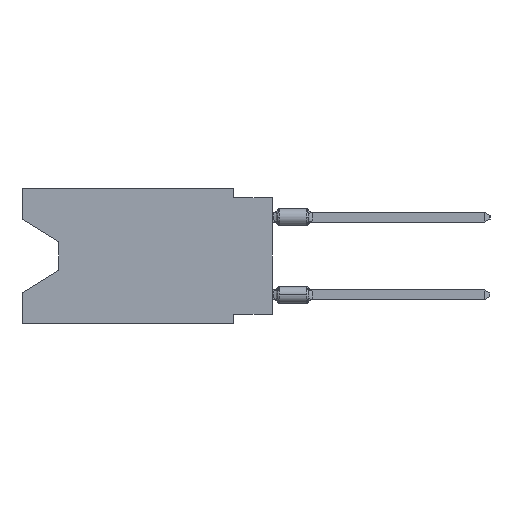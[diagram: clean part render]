
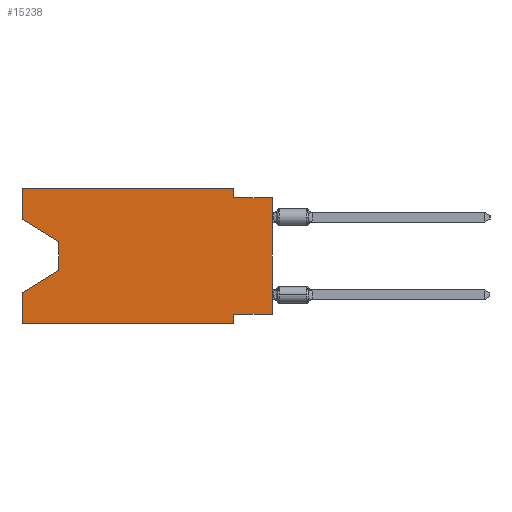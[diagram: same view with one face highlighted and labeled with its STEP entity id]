
A CAD part, left-side view. The second image highlights one B-rep face of the part: STEP entity #15238.
In plain terms, the highlighted planar face has unit normal (-1, 0, 0).
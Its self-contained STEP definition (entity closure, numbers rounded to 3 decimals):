
#45 = CARTESIAN_POINT ( 'NONE',  ( 0., 16.383, 0. ) ) ;
#332 = LINE ( 'NONE', #27026, #490 ) ;
#490 = VECTOR ( 'NONE', #9860, 1000. ) ;
#760 = LINE ( 'NONE', #24597, #28645 ) ;
#1289 = DIRECTION ( 'NONE',  ( 0., -1., 0. ) ) ;
#1297 = VERTEX_POINT ( 'NONE', #8697 ) ;
#1595 = VERTEX_POINT ( 'NONE', #38771 ) ;
#2137 = CARTESIAN_POINT ( 'NONE',  ( 0., 2.54, -8.255 ) ) ;
#2573 = CARTESIAN_POINT ( 'NONE',  ( 0., 13.97, -3.505 ) ) ;
#2845 = EDGE_CURVE ( 'NONE', #24659, #15315, #19701, .T. ) ;
#3025 = DIRECTION ( 'NONE',  ( 0., 0., -1. ) ) ;
#3089 = AXIS2_PLACEMENT_3D ( 'NONE', #24086, #35317, #35539 ) ;
#3456 = ORIENTED_EDGE ( 'NONE', *, *, #19535, .F. ) ;
#3770 = EDGE_CURVE ( 'NONE', #29179, #15438, #28656, .T. ) ;
#4146 = VERTEX_POINT ( 'NONE', #2573 ) ;
#4383 = ORIENTED_EDGE ( 'NONE', *, *, #30460, .F. ) ;
#5077 = FACE_OUTER_BOUND ( 'NONE', #12166, .T. ) ;
#5600 = CARTESIAN_POINT ( 'NONE',  ( 0., 0., 0. ) ) ;
#5640 = EDGE_CURVE ( 'NONE', #15473, #15072, #760, .T. ) ;
#5659 = VECTOR ( 'NONE', #24197, 1000. ) ;
#6470 = ORIENTED_EDGE ( 'NONE', *, *, #36871, .F. ) ;
#6519 = CARTESIAN_POINT ( 'NONE',  ( 0., 13.97, -5.385 ) ) ;
#7117 = VERTEX_POINT ( 'NONE', #41844 ) ;
#7897 = LINE ( 'NONE', #42127, #26579 ) ;
#8697 = CARTESIAN_POINT ( 'NONE',  ( 0., 0., -0.635 ) ) ;
#9201 = EDGE_CURVE ( 'NONE', #7117, #1297, #18195, .T. ) ;
#9860 = DIRECTION ( 'NONE',  ( 0., -1., 0. ) ) ;
#10411 = ORIENTED_EDGE ( 'NONE', *, *, #14484, .F. ) ;
#10516 = CARTESIAN_POINT ( 'NONE',  ( 0., 0., -8.255 ) ) ;
#10759 = CARTESIAN_POINT ( 'NONE',  ( 0., 16.383, -2.038 ) ) ;
#10935 = DIRECTION ( 'NONE',  ( 0., -1., 0. ) ) ;
#11017 = CARTESIAN_POINT ( 'NONE',  ( 0., 16.383, -8.89 ) ) ;
#12166 = EDGE_LOOP ( 'NONE', ( #20051, #15678, #16820, #41837, #31836, #3456, #4383, #42537, #16226, #40885, #10411, #6470 ) ) ;
#13141 = CARTESIAN_POINT ( 'NONE',  ( 0., 16.383, 0. ) ) ;
#14484 = EDGE_CURVE ( 'NONE', #18626, #24659, #7897, .T. ) ;
#14534 = VECTOR ( 'NONE', #32481, 1000. ) ;
#15072 = VERTEX_POINT ( 'NONE', #17059 ) ;
#15238 = ADVANCED_FACE ( 'NONE', ( #5077 ), #32442, .F. ) ;
#15315 = VERTEX_POINT ( 'NONE', #26036 ) ;
#15438 = VERTEX_POINT ( 'NONE', #39933 ) ;
#15473 = VERTEX_POINT ( 'NONE', #11017 ) ;
#15678 = ORIENTED_EDGE ( 'NONE', *, *, #30527, .T. ) ;
#15765 = CARTESIAN_POINT ( 'NONE',  ( 0., 2.54, 0. ) ) ;
#16226 = ORIENTED_EDGE ( 'NONE', *, *, #38185, .F. ) ;
#16489 = CARTESIAN_POINT ( 'NONE',  ( 0., 13.97, -3.505 ) ) ;
#16645 = CARTESIAN_POINT ( 'NONE',  ( 0., 2.54, -8.89 ) ) ;
#16820 = ORIENTED_EDGE ( 'NONE', *, *, #3770, .T. ) ;
#17059 = CARTESIAN_POINT ( 'NONE',  ( 0., 2.54, -8.89 ) ) ;
#18195 = LINE ( 'NONE', #5600, #35931 ) ;
#18626 = VERTEX_POINT ( 'NONE', #13141 ) ;
#18634 = VECTOR ( 'NONE', #31296, 1000. ) ;
#18746 = VECTOR ( 'NONE', #23951, 1000. ) ;
#19535 = EDGE_CURVE ( 'NONE', #25486, #15072, #26563, .T. ) ;
#19701 = LINE ( 'NONE', #20352, #23589 ) ;
#20051 = ORIENTED_EDGE ( 'NONE', *, *, #24653, .T. ) ;
#20352 = CARTESIAN_POINT ( 'NONE',  ( 0., 2.54, 0. ) ) ;
#21167 = CARTESIAN_POINT ( 'NONE',  ( 0., 13.97, -5.385 ) ) ;
#22773 = VECTOR ( 'NONE', #23230, 1000. ) ;
#23230 = DIRECTION ( 'NONE',  ( 0., 0., 1. ) ) ;
#23589 = VECTOR ( 'NONE', #40641, 1000. ) ;
#23621 = VECTOR ( 'NONE', #3025, 1000. ) ;
#23951 = DIRECTION ( 'NONE',  ( 0., 1., 0. ) ) ;
#23981 = LINE ( 'NONE', #10759, #5659 ) ;
#24086 = CARTESIAN_POINT ( 'NONE',  ( 0., 16.383, 0. ) ) ;
#24197 = DIRECTION ( 'NONE',  ( 0., -0.855, -0.519 ) ) ;
#24597 = CARTESIAN_POINT ( 'NONE',  ( 0., 16.383, -8.89 ) ) ;
#24653 = EDGE_CURVE ( 'NONE', #1595, #4146, #23981, .T. ) ;
#24659 = VERTEX_POINT ( 'NONE', #15765 ) ;
#25486 = VERTEX_POINT ( 'NONE', #2137 ) ;
#26036 = CARTESIAN_POINT ( 'NONE',  ( 0., 2.54, -0.635 ) ) ;
#26563 = LINE ( 'NONE', #16645, #14534 ) ;
#26579 = VECTOR ( 'NONE', #1289, 1000. ) ;
#27026 = CARTESIAN_POINT ( 'NONE',  ( 0., 0., -0.635 ) ) ;
#28645 = VECTOR ( 'NONE', #10935, 1000. ) ;
#28656 = LINE ( 'NONE', #21167, #18634 ) ;
#29179 = VERTEX_POINT ( 'NONE', #6519 ) ;
#29699 = LINE ( 'NONE', #40494, #36868 ) ;
#30460 = EDGE_CURVE ( 'NONE', #7117, #25486, #34125, .T. ) ;
#30527 = EDGE_CURVE ( 'NONE', #4146, #29179, #33257, .T. ) ;
#31296 = DIRECTION ( 'NONE',  ( 0., 0.855, -0.519 ) ) ;
#31836 = ORIENTED_EDGE ( 'NONE', *, *, #5640, .T. ) ;
#32442 = PLANE ( 'NONE',  #3089 ) ;
#32481 = DIRECTION ( 'NONE',  ( 0., 0., -1. ) ) ;
#32969 = LINE ( 'NONE', #45, #22773 ) ;
#33257 = LINE ( 'NONE', #16489, #23621 ) ;
#33675 = DIRECTION ( 'NONE',  ( 0., 0., 1. ) ) ;
#34125 = LINE ( 'NONE', #10516, #18746 ) ;
#35317 = DIRECTION ( 'NONE',  ( 1., 0., 0. ) ) ;
#35539 = DIRECTION ( 'NONE',  ( 0., 0., -1. ) ) ;
#35931 = VECTOR ( 'NONE', #38705, 1000. ) ;
#36436 = EDGE_CURVE ( 'NONE', #15473, #15438, #29699, .T. ) ;
#36868 = VECTOR ( 'NONE', #33675, 1000. ) ;
#36871 = EDGE_CURVE ( 'NONE', #1595, #18626, #32969, .T. ) ;
#38185 = EDGE_CURVE ( 'NONE', #15315, #1297, #332, .T. ) ;
#38705 = DIRECTION ( 'NONE',  ( 0., 0., 1. ) ) ;
#38771 = CARTESIAN_POINT ( 'NONE',  ( 0., 16.383, -2.038 ) ) ;
#39933 = CARTESIAN_POINT ( 'NONE',  ( 0., 16.383, -6.852 ) ) ;
#40494 = CARTESIAN_POINT ( 'NONE',  ( 0., 16.383, 0. ) ) ;
#40641 = DIRECTION ( 'NONE',  ( 0., 0., -1. ) ) ;
#40885 = ORIENTED_EDGE ( 'NONE', *, *, #2845, .F. ) ;
#41837 = ORIENTED_EDGE ( 'NONE', *, *, #36436, .F. ) ;
#41844 = CARTESIAN_POINT ( 'NONE',  ( 0., 0., -8.255 ) ) ;
#42127 = CARTESIAN_POINT ( 'NONE',  ( 0., 16.383, 0. ) ) ;
#42537 = ORIENTED_EDGE ( 'NONE', *, *, #9201, .T. ) ;
